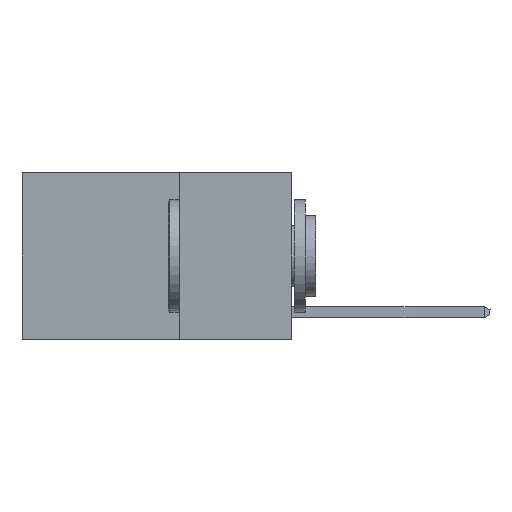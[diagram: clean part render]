
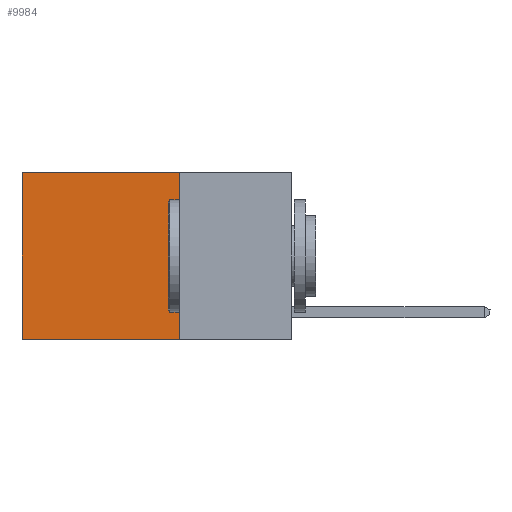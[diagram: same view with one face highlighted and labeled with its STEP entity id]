
A CAD part, left-side view. The second image highlights one B-rep face of the part: STEP entity #9984.
In plain terms, the highlighted planar face has unit normal (-1, 0, 0).
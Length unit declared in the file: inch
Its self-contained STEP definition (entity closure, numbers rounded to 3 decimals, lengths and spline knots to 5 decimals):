
#17 = CARTESIAN_POINT ( 'NONE',  ( 0.2625, 0.6, 0. ) ) ;
#201 = EDGE_LOOP ( 'NONE', ( #13357, #6209, #9579, #14293 ) ) ;
#288 = CARTESIAN_POINT ( 'NONE',  ( 0.2625, 0.25, -0.37 ) ) ;
#290 = LINE ( 'NONE', #5927, #3037 ) ;
#661 = CARTESIAN_POINT ( 'NONE',  ( 0.2625, 0.6, -0.37 ) ) ;
#2143 = DIRECTION ( 'NONE',  ( 0., 0., -1. ) ) ;
#2345 = CARTESIAN_POINT ( 'NONE',  ( 0.2625, 0.25, 0. ) ) ;
#2370 = CARTESIAN_POINT ( 'NONE',  ( 0.2625, 0.25, 0. ) ) ;
#2381 = EDGE_CURVE ( 'NONE', #11928, #8743, #3971, .T. ) ;
#2671 = DIRECTION ( 'NONE',  ( 0., 1., 0. ) ) ;
#2978 = VECTOR ( 'NONE', #4660, 39.37008 ) ;
#3037 = VECTOR ( 'NONE', #2671, 39.37008 ) ;
#3398 = DIRECTION ( 'NONE',  ( 1., 0., 0. ) ) ;
#3971 = LINE ( 'NONE', #10235, #11887 ) ;
#4323 = DIRECTION ( 'NONE',  ( 0., 1., 0. ) ) ;
#4660 = DIRECTION ( 'NONE',  ( 0., 0., -1. ) ) ;
#5455 = AXIS2_PLACEMENT_3D ( 'NONE', #2345, #3398, #2143 ) ;
#5584 = CARTESIAN_POINT ( 'NONE',  ( 0.2625, 0.25, -0.37 ) ) ;
#5927 = CARTESIAN_POINT ( 'NONE',  ( 0.2625, 0.25, 0. ) ) ;
#6209 = ORIENTED_EDGE ( 'NONE', *, *, #12249, .F. ) ;
#6565 = EDGE_CURVE ( 'NONE', #10197, #11928, #290, .T. ) ;
#6820 = LINE ( 'NONE', #5584, #9258 ) ;
#8743 = VERTEX_POINT ( 'NONE', #661 ) ;
#9032 = LINE ( 'NONE', #2370, #2978 ) ;
#9258 = VECTOR ( 'NONE', #4323, 39.37008 ) ;
#9368 = PLANE ( 'NONE',  #5455 ) ;
#9579 = ORIENTED_EDGE ( 'NONE', *, *, #12684, .F. ) ;
#9797 = VERTEX_POINT ( 'NONE', #288 ) ;
#9984 = ADVANCED_FACE ( 'NONE', ( #11132 ), #9368, .F. ) ;
#10197 = VERTEX_POINT ( 'NONE', #14463 ) ;
#10235 = CARTESIAN_POINT ( 'NONE',  ( 0.2625, 0.6, 0. ) ) ;
#10281 = DIRECTION ( 'NONE',  ( 0., 0., -1. ) ) ;
#11132 = FACE_OUTER_BOUND ( 'NONE', #201, .T. ) ;
#11887 = VECTOR ( 'NONE', #10281, 39.37008 ) ;
#11928 = VERTEX_POINT ( 'NONE', #17 ) ;
#12249 = EDGE_CURVE ( 'NONE', #9797, #8743, #6820, .T. ) ;
#12684 = EDGE_CURVE ( 'NONE', #10197, #9797, #9032, .T. ) ;
#13357 = ORIENTED_EDGE ( 'NONE', *, *, #2381, .T. ) ;
#14293 = ORIENTED_EDGE ( 'NONE', *, *, #6565, .T. ) ;
#14463 = CARTESIAN_POINT ( 'NONE',  ( 0.2625, 0.25, 0. ) ) ;
